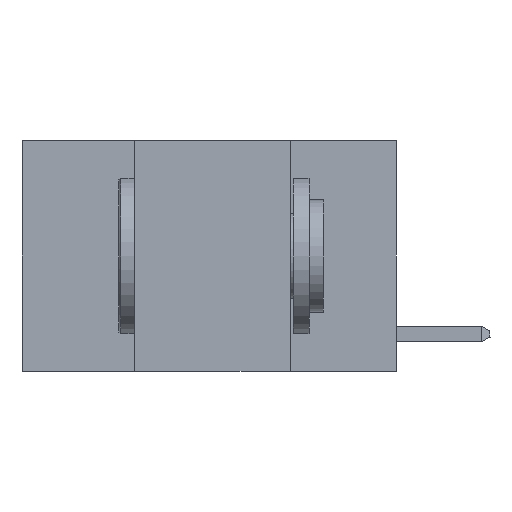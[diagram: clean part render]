
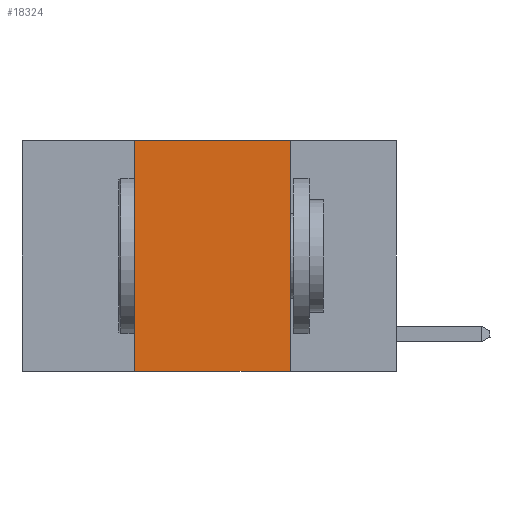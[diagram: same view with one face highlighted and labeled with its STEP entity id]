
A CAD part, left-side view. The second image highlights one B-rep face of the part: STEP entity #18324.
In plain terms, the highlighted planar face has unit normal (-1, 0, 0).
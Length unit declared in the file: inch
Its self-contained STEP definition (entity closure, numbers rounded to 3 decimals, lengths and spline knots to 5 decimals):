
#391 = ORIENTED_EDGE ( 'NONE', *, *, #11359, .T. ) ;
#1185 = CARTESIAN_POINT ( 'NONE',  ( 0., 0.6, -0.37 ) ) ;
#1275 = AXIS2_PLACEMENT_3D ( 'NONE', #5825, #7262, #17181 ) ;
#3402 = ORIENTED_EDGE ( 'NONE', *, *, #18342, .F. ) ;
#3953 = VERTEX_POINT ( 'NONE', #12830 ) ;
#4317 = PLANE ( 'NONE',  #1275 ) ;
#5253 = VECTOR ( 'NONE', #18548, 39.37008 ) ;
#5735 = VERTEX_POINT ( 'NONE', #11855 ) ;
#5783 = VECTOR ( 'NONE', #18543, 39.37008 ) ;
#5825 = CARTESIAN_POINT ( 'NONE',  ( 0., 0.6, 0. ) ) ;
#6463 = VECTOR ( 'NONE', #8542, 39.37008 ) ;
#7065 = CARTESIAN_POINT ( 'NONE',  ( 0., 0.6, 0. ) ) ;
#7262 = DIRECTION ( 'NONE',  ( 1., 0., 0. ) ) ;
#7538 = EDGE_CURVE ( 'NONE', #5735, #12138, #17056, .T. ) ;
#8542 = DIRECTION ( 'NONE',  ( 0., -1., 0. ) ) ;
#8749 = CARTESIAN_POINT ( 'NONE',  ( 0., 0.42, 0. ) ) ;
#9385 = EDGE_LOOP ( 'NONE', ( #3402, #18594, #15306, #391 ) ) ;
#10038 = FACE_OUTER_BOUND ( 'NONE', #9385, .T. ) ;
#10137 = CARTESIAN_POINT ( 'NONE',  ( 0., 0.17, 0. ) ) ;
#10241 = VERTEX_POINT ( 'NONE', #15372 ) ;
#11359 = EDGE_CURVE ( 'NONE', #5735, #3953, #14928, .T. ) ;
#11855 = CARTESIAN_POINT ( 'NONE',  ( 0., 0.42, -0.37 ) ) ;
#12138 = VERTEX_POINT ( 'NONE', #18589 ) ;
#12560 = EDGE_CURVE ( 'NONE', #12138, #10241, #12681, .T. ) ;
#12681 = LINE ( 'NONE', #7065, #16444 ) ;
#12725 = DIRECTION ( 'NONE',  ( 0., -1., 0. ) ) ;
#12830 = CARTESIAN_POINT ( 'NONE',  ( 0., 0.17, -0.37 ) ) ;
#13347 = LINE ( 'NONE', #10137, #5783 ) ;
#14928 = LINE ( 'NONE', #1185, #6463 ) ;
#15306 = ORIENTED_EDGE ( 'NONE', *, *, #7538, .F. ) ;
#15372 = CARTESIAN_POINT ( 'NONE',  ( 0., 0.17, 0. ) ) ;
#16444 = VECTOR ( 'NONE', #12725, 39.37008 ) ;
#17056 = LINE ( 'NONE', #8749, #5253 ) ;
#17181 = DIRECTION ( 'NONE',  ( 0., 0., -1. ) ) ;
#18324 = ADVANCED_FACE ( 'NONE', ( #10038 ), #4317, .F. ) ;
#18342 = EDGE_CURVE ( 'NONE', #10241, #3953, #13347, .T. ) ;
#18543 = DIRECTION ( 'NONE',  ( 0., 0., -1. ) ) ;
#18548 = DIRECTION ( 'NONE',  ( 0., 0., 1. ) ) ;
#18589 = CARTESIAN_POINT ( 'NONE',  ( 0., 0.42, 0. ) ) ;
#18594 = ORIENTED_EDGE ( 'NONE', *, *, #12560, .F. ) ;
